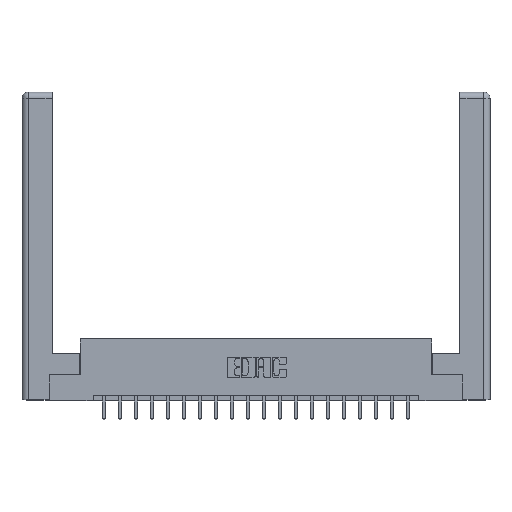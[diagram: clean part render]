
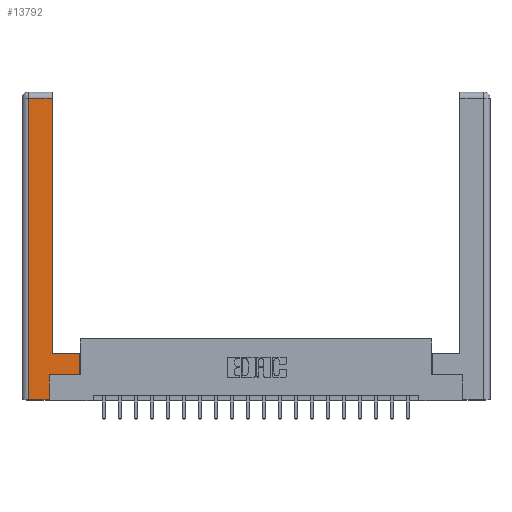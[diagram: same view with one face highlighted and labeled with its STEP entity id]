
A CAD part, top view. The second image highlights one B-rep face of the part: STEP entity #13792.
In plain terms, the highlighted planar face has unit normal (0, 0, 1).
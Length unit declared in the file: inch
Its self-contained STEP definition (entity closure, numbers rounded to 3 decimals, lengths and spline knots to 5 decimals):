
#427 = CARTESIAN_POINT ( 'NONE',  ( 0.565, 0.245, 0. ) ) ;
#624 = LINE ( 'NONE', #4978, #15698 ) ;
#668 = VERTEX_POINT ( 'NONE', #15855 ) ;
#819 = CARTESIAN_POINT ( 'NONE',  ( 0.265, 0., 0. ) ) ;
#1054 = CARTESIAN_POINT ( 'NONE',  ( 0.295, 2.94, 0. ) ) ;
#1229 = DIRECTION ( 'NONE',  ( 0., 1., 0. ) ) ;
#1324 = VECTOR ( 'NONE', #17340, 39.37008 ) ;
#1525 = ORIENTED_EDGE ( 'NONE', *, *, #2830, .T. ) ;
#1635 = EDGE_LOOP ( 'NONE', ( #9150, #18117, #1525, #8056, #19583, #1740, #18098, #6161 ) ) ;
#1740 = ORIENTED_EDGE ( 'NONE', *, *, #18329, .T. ) ;
#1745 = DIRECTION ( 'NONE',  ( -1., 0., 0. ) ) ;
#2665 = LINE ( 'NONE', #12478, #9585 ) ;
#2758 = DIRECTION ( 'NONE',  ( 0., 0., -1. ) ) ;
#2830 = EDGE_CURVE ( 'NONE', #16250, #19278, #14648, .T. ) ;
#2843 = LINE ( 'NONE', #18290, #7459 ) ;
#3335 = DIRECTION ( 'NONE',  ( 0., -1., 0. ) ) ;
#3341 = CARTESIAN_POINT ( 'NONE',  ( 0.295, 0.45, 0. ) ) ;
#3639 = VERTEX_POINT ( 'NONE', #819 ) ;
#4829 = CARTESIAN_POINT ( 'NONE',  ( 0.0615, 0., 0. ) ) ;
#4898 = EDGE_CURVE ( 'NONE', #3639, #668, #17389, .T. ) ;
#4978 = CARTESIAN_POINT ( 'NONE',  ( 0.295, 3., 0. ) ) ;
#5378 = CARTESIAN_POINT ( 'NONE',  ( 0.565, 0.45, 0. ) ) ;
#5578 = DIRECTION ( 'NONE',  ( 1., 0., 0. ) ) ;
#5964 = CARTESIAN_POINT ( 'NONE',  ( 0.295, 0.45, 0. ) ) ;
#6074 = CARTESIAN_POINT ( 'NONE',  ( 0.265, 0.245, 0. ) ) ;
#6161 = ORIENTED_EDGE ( 'NONE', *, *, #16509, .T. ) ;
#7459 = VECTOR ( 'NONE', #1745, 39.37008 ) ;
#8056 = ORIENTED_EDGE ( 'NONE', *, *, #11644, .T. ) ;
#8343 = LINE ( 'NONE', #15537, #11965 ) ;
#8363 = VERTEX_POINT ( 'NONE', #427 ) ;
#9150 = ORIENTED_EDGE ( 'NONE', *, *, #15337, .T. ) ;
#9585 = VECTOR ( 'NONE', #15816, 39.37008 ) ;
#9786 = CARTESIAN_POINT ( 'NONE',  ( 0.0615, 0., 0. ) ) ;
#10459 = EDGE_CURVE ( 'NONE', #8363, #11203, #2665, .T. ) ;
#10514 = FACE_OUTER_BOUND ( 'NONE', #1635, .T. ) ;
#10767 = VERTEX_POINT ( 'NONE', #3341 ) ;
#10983 = VERTEX_POINT ( 'NONE', #1054 ) ;
#11203 = VERTEX_POINT ( 'NONE', #5378 ) ;
#11644 = EDGE_CURVE ( 'NONE', #19278, #3639, #8343, .T. ) ;
#11855 = VECTOR ( 'NONE', #3335, 39.37008 ) ;
#11965 = VECTOR ( 'NONE', #5578, 39.37008 ) ;
#12246 = CARTESIAN_POINT ( 'NONE',  ( 0.0615, 2.94, 0. ) ) ;
#12478 = CARTESIAN_POINT ( 'NONE',  ( 0.565, 0.45, 0. ) ) ;
#12571 = DIRECTION ( 'NONE',  ( -1., 0., 0. ) ) ;
#13375 = EDGE_CURVE ( 'NONE', #10983, #16250, #2843, .T. ) ;
#13792 = ADVANCED_FACE ( 'NONE', ( #10514 ), #15781, .F. ) ;
#14648 = LINE ( 'NONE', #4829, #11855 ) ;
#14737 = DIRECTION ( 'NONE',  ( 0., 1., 0. ) ) ;
#15337 = EDGE_CURVE ( 'NONE', #10767, #10983, #624, .T. ) ;
#15537 = CARTESIAN_POINT ( 'NONE',  ( 0.265, 0., 0. ) ) ;
#15698 = VECTOR ( 'NONE', #14737, 39.37008 ) ;
#15781 = PLANE ( 'NONE',  #19535 ) ;
#15816 = DIRECTION ( 'NONE',  ( 0., 1., 0. ) ) ;
#15855 = CARTESIAN_POINT ( 'NONE',  ( 0.265, 0.245, 0. ) ) ;
#16250 = VERTEX_POINT ( 'NONE', #12246 ) ;
#16509 = EDGE_CURVE ( 'NONE', #11203, #10767, #19720, .T. ) ;
#17049 = CARTESIAN_POINT ( 'NONE',  ( 0.565, 0.245, 0. ) ) ;
#17340 = DIRECTION ( 'NONE',  ( -1., 0., 0. ) ) ;
#17389 = LINE ( 'NONE', #6074, #17897 ) ;
#17506 = VECTOR ( 'NONE', #18466, 39.37008 ) ;
#17897 = VECTOR ( 'NONE', #1229, 39.37008 ) ;
#18098 = ORIENTED_EDGE ( 'NONE', *, *, #10459, .T. ) ;
#18117 = ORIENTED_EDGE ( 'NONE', *, *, #13375, .T. ) ;
#18239 = LINE ( 'NONE', #17049, #17506 ) ;
#18290 = CARTESIAN_POINT ( 'NONE',  ( 0.0615, 2.94, 0. ) ) ;
#18329 = EDGE_CURVE ( 'NONE', #668, #8363, #18239, .T. ) ;
#18466 = DIRECTION ( 'NONE',  ( 1., 0., 0. ) ) ;
#19278 = VERTEX_POINT ( 'NONE', #9786 ) ;
#19535 = AXIS2_PLACEMENT_3D ( 'NONE', #20687, #2758, #12571 ) ;
#19583 = ORIENTED_EDGE ( 'NONE', *, *, #4898, .T. ) ;
#19720 = LINE ( 'NONE', #5964, #1324 ) ;
#20687 = CARTESIAN_POINT ( 'NONE',  ( 0., 0., 0. ) ) ;
